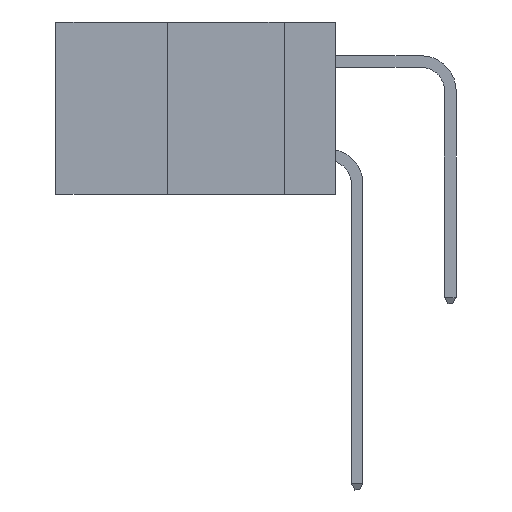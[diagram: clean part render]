
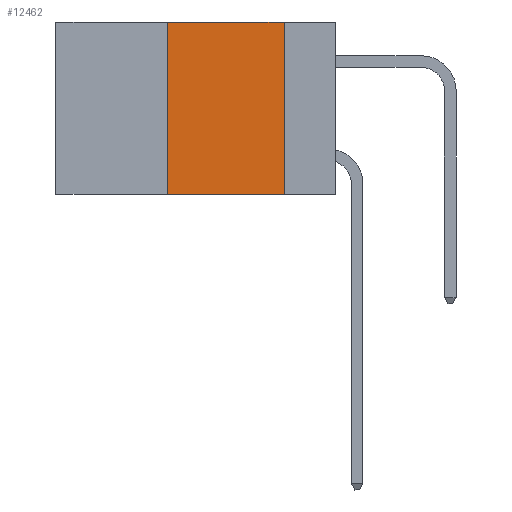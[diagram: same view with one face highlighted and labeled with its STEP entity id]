
A CAD part, left-side view. The second image highlights one B-rep face of the part: STEP entity #12462.
In plain terms, the highlighted planar face has unit normal (-1, 0, 0).
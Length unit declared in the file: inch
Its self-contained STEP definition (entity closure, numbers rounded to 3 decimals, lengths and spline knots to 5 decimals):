
#1114 = DIRECTION ( 'NONE',  ( 0., -1., 0. ) ) ;
#1260 = CARTESIAN_POINT ( 'NONE',  ( 0., 0.6, 0. ) ) ;
#1475 = VECTOR ( 'NONE', #20132, 39.37008 ) ;
#1706 = CARTESIAN_POINT ( 'NONE',  ( 0., 0.6, -0.37 ) ) ;
#2336 = DIRECTION ( 'NONE',  ( 1., 0., 0. ) ) ;
#4028 = LINE ( 'NONE', #1706, #12158 ) ;
#6051 = CARTESIAN_POINT ( 'NONE',  ( 0., 0.36, 0. ) ) ;
#7391 = LINE ( 'NONE', #30595, #1475 ) ;
#9950 = VECTOR ( 'NONE', #1114, 39.37008 ) ;
#10349 = VECTOR ( 'NONE', #33592, 39.37008 ) ;
#12158 = VECTOR ( 'NONE', #32544, 39.37008 ) ;
#12462 = ADVANCED_FACE ( 'NONE', ( #21561 ), #16549, .F. ) ;
#14105 = CARTESIAN_POINT ( 'NONE',  ( 0., 0.36, -0.37 ) ) ;
#15282 = AXIS2_PLACEMENT_3D ( 'NONE', #16699, #2336, #40795 ) ;
#15598 = VERTEX_POINT ( 'NONE', #14105 ) ;
#16136 = CARTESIAN_POINT ( 'NONE',  ( 0., 0.11, 0. ) ) ;
#16549 = PLANE ( 'NONE',  #15282 ) ;
#16699 = CARTESIAN_POINT ( 'NONE',  ( 0., 0.6, 0. ) ) ;
#17560 = ORIENTED_EDGE ( 'NONE', *, *, #35760, .T. ) ;
#18090 = VERTEX_POINT ( 'NONE', #16136 ) ;
#18694 = EDGE_CURVE ( 'NONE', #25451, #18090, #42680, .T. ) ;
#19635 = LINE ( 'NONE', #6051, #10349 ) ;
#20111 = EDGE_CURVE ( 'NONE', #15598, #25451, #19635, .T. ) ;
#20132 = DIRECTION ( 'NONE',  ( 0., 0., -1. ) ) ;
#21561 = FACE_OUTER_BOUND ( 'NONE', #43473, .T. ) ;
#25451 = VERTEX_POINT ( 'NONE', #28721 ) ;
#26432 = VERTEX_POINT ( 'NONE', #31070 ) ;
#28721 = CARTESIAN_POINT ( 'NONE',  ( 0., 0.36, 0. ) ) ;
#30595 = CARTESIAN_POINT ( 'NONE',  ( 0., 0.11, 0. ) ) ;
#31070 = CARTESIAN_POINT ( 'NONE',  ( 0., 0.11, -0.37 ) ) ;
#32544 = DIRECTION ( 'NONE',  ( 0., -1., 0. ) ) ;
#33498 = ORIENTED_EDGE ( 'NONE', *, *, #20111, .F. ) ;
#33592 = DIRECTION ( 'NONE',  ( 0., 0., 1. ) ) ;
#35760 = EDGE_CURVE ( 'NONE', #15598, #26432, #4028, .T. ) ;
#39873 = EDGE_CURVE ( 'NONE', #18090, #26432, #7391, .T. ) ;
#40470 = ORIENTED_EDGE ( 'NONE', *, *, #39873, .F. ) ;
#40795 = DIRECTION ( 'NONE',  ( 0., 0., -1. ) ) ;
#42680 = LINE ( 'NONE', #1260, #9950 ) ;
#43473 = EDGE_LOOP ( 'NONE', ( #40470, #43607, #33498, #17560 ) ) ;
#43607 = ORIENTED_EDGE ( 'NONE', *, *, #18694, .F. ) ;
